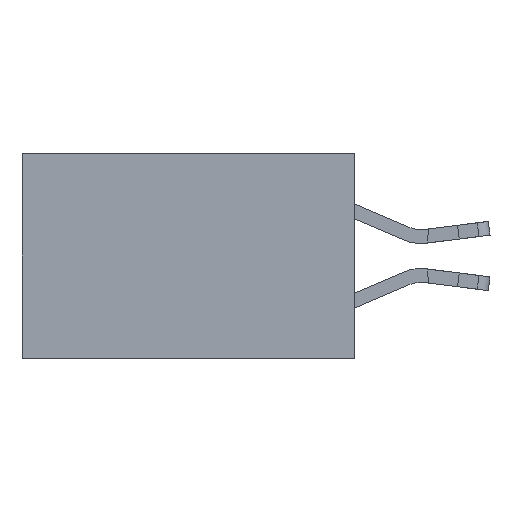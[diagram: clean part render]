
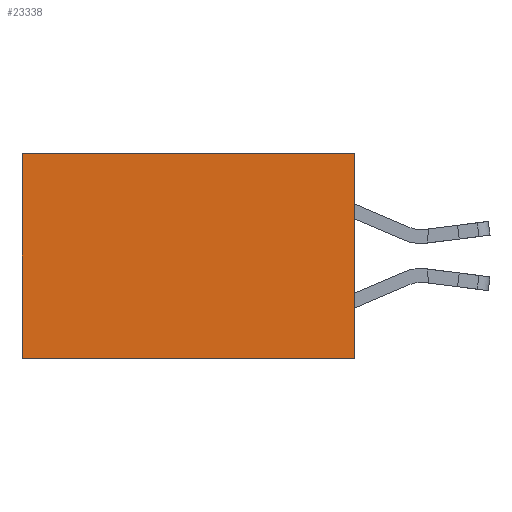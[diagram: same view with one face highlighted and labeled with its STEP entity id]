
A CAD part, left-side view. The second image highlights one B-rep face of the part: STEP entity #23338.
In plain terms, the highlighted planar face has unit normal (-1, 0, 0).
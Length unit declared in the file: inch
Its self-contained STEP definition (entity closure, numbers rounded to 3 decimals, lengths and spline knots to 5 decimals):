
#373 = EDGE_CURVE ( 'NONE', #22154, #22362, #19970, .T. ) ;
#945 = CARTESIAN_POINT ( 'NONE',  ( 0.298, 0., -0.37 ) ) ;
#2505 = LINE ( 'NONE', #21031, #8491 ) ;
#3002 = EDGE_LOOP ( 'NONE', ( #20856, #10802, #20875, #15526 ) ) ;
#3220 = DIRECTION ( 'NONE',  ( 0., 1., 0. ) ) ;
#3855 = EDGE_CURVE ( 'NONE', #13565, #11651, #5536, .T. ) ;
#4767 = AXIS2_PLACEMENT_3D ( 'NONE', #7334, #9548, #24531 ) ;
#5536 = LINE ( 'NONE', #7165, #15793 ) ;
#7165 = CARTESIAN_POINT ( 'NONE',  ( 0.298, 0., -0.37 ) ) ;
#7334 = CARTESIAN_POINT ( 'NONE',  ( 0.298, 0., 0. ) ) ;
#8464 = FACE_OUTER_BOUND ( 'NONE', #3002, .T. ) ;
#8491 = VECTOR ( 'NONE', #25315, 39.37008 ) ;
#9548 = DIRECTION ( 'NONE',  ( 1., 0., 0. ) ) ;
#10802 = ORIENTED_EDGE ( 'NONE', *, *, #3855, .F. ) ;
#11651 = VERTEX_POINT ( 'NONE', #18482 ) ;
#11886 = EDGE_CURVE ( 'NONE', #22154, #13565, #22705, .T. ) ;
#13565 = VERTEX_POINT ( 'NONE', #945 ) ;
#14287 = VECTOR ( 'NONE', #25938, 39.37008 ) ;
#15526 = ORIENTED_EDGE ( 'NONE', *, *, #373, .T. ) ;
#15793 = VECTOR ( 'NONE', #3220, 39.37008 ) ;
#16403 = VECTOR ( 'NONE', #25538, 39.37008 ) ;
#18349 = CARTESIAN_POINT ( 'NONE',  ( 0.298, 0., 0. ) ) ;
#18482 = CARTESIAN_POINT ( 'NONE',  ( 0.298, 0.6, -0.37 ) ) ;
#19970 = LINE ( 'NONE', #26035, #14287 ) ;
#20254 = PLANE ( 'NONE',  #4767 ) ;
#20856 = ORIENTED_EDGE ( 'NONE', *, *, #22923, .T. ) ;
#20875 = ORIENTED_EDGE ( 'NONE', *, *, #11886, .F. ) ;
#21031 = CARTESIAN_POINT ( 'NONE',  ( 0.298, 0.6, 0. ) ) ;
#21492 = CARTESIAN_POINT ( 'NONE',  ( 0.298, 0.6, 0. ) ) ;
#22154 = VERTEX_POINT ( 'NONE', #18349 ) ;
#22362 = VERTEX_POINT ( 'NONE', #21492 ) ;
#22705 = LINE ( 'NONE', #27758, #16403 ) ;
#22923 = EDGE_CURVE ( 'NONE', #22362, #11651, #2505, .T. ) ;
#23338 = ADVANCED_FACE ( 'NONE', ( #8464 ), #20254, .F. ) ;
#24531 = DIRECTION ( 'NONE',  ( 0., 0., -1. ) ) ;
#25315 = DIRECTION ( 'NONE',  ( 0., 0., -1. ) ) ;
#25538 = DIRECTION ( 'NONE',  ( 0., 0., -1. ) ) ;
#25938 = DIRECTION ( 'NONE',  ( 0., 1., 0. ) ) ;
#26035 = CARTESIAN_POINT ( 'NONE',  ( 0.298, 0., 0. ) ) ;
#27758 = CARTESIAN_POINT ( 'NONE',  ( 0.298, 0., 0. ) ) ;
